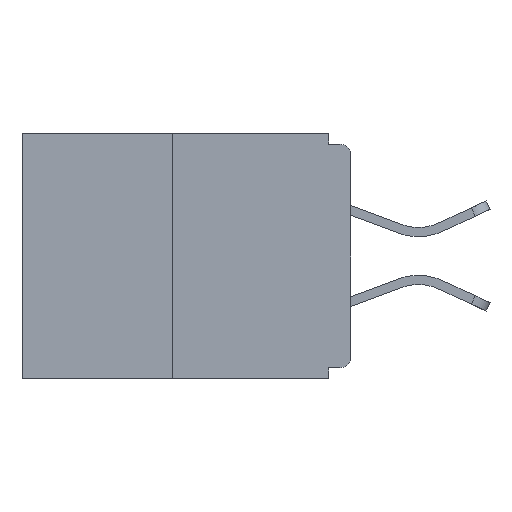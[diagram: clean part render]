
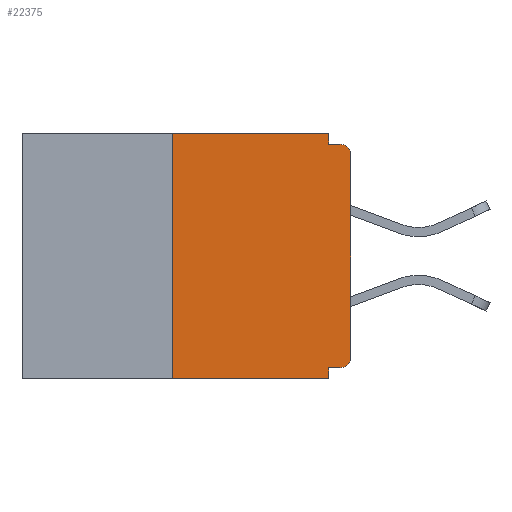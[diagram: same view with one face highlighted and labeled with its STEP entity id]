
A CAD part, left-side view. The second image highlights one B-rep face of the part: STEP entity #22375.
In plain terms, the highlighted planar face has unit normal (-1, 0, 0).
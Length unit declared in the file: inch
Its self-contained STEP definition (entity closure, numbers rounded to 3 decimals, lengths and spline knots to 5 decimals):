
#107 = DIRECTION ( 'NONE',  ( 0., -1., 0. ) ) ;
#208 = VERTEX_POINT ( 'NONE', #11022 ) ;
#245 = CARTESIAN_POINT ( 'NONE',  ( 0., 0.46, 0. ) ) ;
#309 = VERTEX_POINT ( 'NONE', #4111 ) ;
#477 = VECTOR ( 'NONE', #15684, 39.37008 ) ;
#879 = EDGE_CURVE ( 'NONE', #23807, #12587, #21511, .T. ) ;
#1698 = ORIENTED_EDGE ( 'NONE', *, *, #21080, .F. ) ;
#1701 = EDGE_CURVE ( 'NONE', #12587, #208, #19088, .T. ) ;
#1755 = VERTEX_POINT ( 'NONE', #23394 ) ;
#2341 = ORIENTED_EDGE ( 'NONE', *, *, #12382, .T. ) ;
#2353 = ORIENTED_EDGE ( 'NONE', *, *, #879, .T. ) ;
#2946 = VERTEX_POINT ( 'NONE', #4518 ) ;
#3126 = DIRECTION ( 'NONE',  ( 0., 0., -1. ) ) ;
#3643 = EDGE_CURVE ( 'NONE', #1755, #23119, #19013, .T. ) ;
#4021 = PLANE ( 'NONE',  #9224 ) ;
#4111 = CARTESIAN_POINT ( 'NONE',  ( 0., 0.25, -0.343 ) ) ;
#4428 = CARTESIAN_POINT ( 'NONE',  ( 0., 0.031, -0.015 ) ) ;
#4518 = CARTESIAN_POINT ( 'NONE',  ( 0., 0.031, -0.343 ) ) ;
#4547 = LINE ( 'NONE', #16645, #14903 ) ;
#4851 = DIRECTION ( 'NONE',  ( 0., 0., -1. ) ) ;
#5368 = VERTEX_POINT ( 'NONE', #4428 ) ;
#6048 = CARTESIAN_POINT ( 'NONE',  ( 0., 0.25, 0. ) ) ;
#6326 = ORIENTED_EDGE ( 'NONE', *, *, #9831, .T. ) ;
#6341 = CARTESIAN_POINT ( 'NONE',  ( 0., 0., -0.03 ) ) ;
#6537 = CARTESIAN_POINT ( 'NONE',  ( 0., 0.031, 0. ) ) ;
#6551 = CARTESIAN_POINT ( 'NONE',  ( 0., 0., 0. ) ) ;
#6879 = DIRECTION ( 'NONE',  ( 0., -1., 0. ) ) ;
#7056 = CARTESIAN_POINT ( 'NONE',  ( 0., 0.46, 0. ) ) ;
#7343 = FACE_OUTER_BOUND ( 'NONE', #18500, .T. ) ;
#8139 = CARTESIAN_POINT ( 'NONE',  ( 0., 0.015, -0.313 ) ) ;
#8490 = DIRECTION ( 'NONE',  ( 0., 1., 0. ) ) ;
#8572 = VECTOR ( 'NONE', #19128, 39.37008 ) ;
#8754 = DIRECTION ( 'NONE',  ( -1., 0., 0. ) ) ;
#8869 = ORIENTED_EDGE ( 'NONE', *, *, #17056, .F. ) ;
#9224 = AXIS2_PLACEMENT_3D ( 'NONE', #245, #20539, #13242 ) ;
#9308 = CARTESIAN_POINT ( 'NONE',  ( 0., 0.031, -0.343 ) ) ;
#9388 = VECTOR ( 'NONE', #18933, 39.37008 ) ;
#9685 = LINE ( 'NONE', #6048, #9388 ) ;
#9831 = EDGE_CURVE ( 'NONE', #1755, #23807, #16474, .T. ) ;
#10270 = CARTESIAN_POINT ( 'NONE',  ( 0., 0., -0.015 ) ) ;
#10283 = LINE ( 'NONE', #7056, #17644 ) ;
#11022 = CARTESIAN_POINT ( 'NONE',  ( 0., 0.015, -0.015 ) ) ;
#12271 = LINE ( 'NONE', #22230, #19795 ) ;
#12316 = DIRECTION ( 'NONE',  ( -1., 0., 0. ) ) ;
#12356 = ORIENTED_EDGE ( 'NONE', *, *, #14428, .F. ) ;
#12382 = EDGE_CURVE ( 'NONE', #309, #2946, #4547, .T. ) ;
#12587 = VERTEX_POINT ( 'NONE', #6341 ) ;
#13242 = DIRECTION ( 'NONE',  ( 0., 0., -1. ) ) ;
#14252 = LINE ( 'NONE', #10270, #477 ) ;
#14428 = EDGE_CURVE ( 'NONE', #23434, #15164, #10283, .T. ) ;
#14903 = VECTOR ( 'NONE', #107, 39.37008 ) ;
#15164 = VERTEX_POINT ( 'NONE', #6537 ) ;
#15374 = LINE ( 'NONE', #9308, #23443 ) ;
#15529 = CARTESIAN_POINT ( 'NONE',  ( 0., 0., -0.313 ) ) ;
#15684 = DIRECTION ( 'NONE',  ( 0., -1., 0. ) ) ;
#15887 = ORIENTED_EDGE ( 'NONE', *, *, #16235, .F. ) ;
#16235 = EDGE_CURVE ( 'NONE', #309, #23434, #9685, .T. ) ;
#16474 = CIRCLE ( 'NONE', #18007, 0.015 ) ;
#16645 = CARTESIAN_POINT ( 'NONE',  ( 0., 0.46, -0.343 ) ) ;
#17056 = EDGE_CURVE ( 'NONE', #5368, #208, #14252, .T. ) ;
#17334 = ORIENTED_EDGE ( 'NONE', *, *, #1701, .T. ) ;
#17565 = CARTESIAN_POINT ( 'NONE',  ( 0., 0.031, -0.328 ) ) ;
#17644 = VECTOR ( 'NONE', #6879, 39.37008 ) ;
#17996 = EDGE_CURVE ( 'NONE', #23119, #2946, #15374, .T. ) ;
#18007 = AXIS2_PLACEMENT_3D ( 'NONE', #8139, #12316, #4851 ) ;
#18066 = CARTESIAN_POINT ( 'NONE',  ( 0., 0.015, -0.03 ) ) ;
#18443 = DIRECTION ( 'NONE',  ( 0., 0., -1. ) ) ;
#18500 = EDGE_LOOP ( 'NONE', ( #12356, #15887, #2341, #21942, #20864, #6326, #2353, #17334, #8869, #1698 ) ) ;
#18933 = DIRECTION ( 'NONE',  ( 0., 0., 1. ) ) ;
#18946 = DIRECTION ( 'NONE',  ( 0., 0., -1. ) ) ;
#19013 = LINE ( 'NONE', #19506, #21586 ) ;
#19088 = CIRCLE ( 'NONE', #23761, 0.015 ) ;
#19128 = DIRECTION ( 'NONE',  ( 0., 0., 1. ) ) ;
#19506 = CARTESIAN_POINT ( 'NONE',  ( 0., 0., -0.328 ) ) ;
#19795 = VECTOR ( 'NONE', #18443, 39.37008 ) ;
#20539 = DIRECTION ( 'NONE',  ( 1., 0., 0. ) ) ;
#20864 = ORIENTED_EDGE ( 'NONE', *, *, #3643, .F. ) ;
#21080 = EDGE_CURVE ( 'NONE', #15164, #5368, #12271, .T. ) ;
#21511 = LINE ( 'NONE', #6551, #8572 ) ;
#21586 = VECTOR ( 'NONE', #8490, 39.37008 ) ;
#21916 = CARTESIAN_POINT ( 'NONE',  ( 0., 0.25, 0. ) ) ;
#21942 = ORIENTED_EDGE ( 'NONE', *, *, #17996, .F. ) ;
#22230 = CARTESIAN_POINT ( 'NONE',  ( 0., 0.031, 0. ) ) ;
#22375 = ADVANCED_FACE ( 'NONE', ( #7343 ), #4021, .F. ) ;
#23119 = VERTEX_POINT ( 'NONE', #17565 ) ;
#23394 = CARTESIAN_POINT ( 'NONE',  ( 0., 0.015, -0.328 ) ) ;
#23434 = VERTEX_POINT ( 'NONE', #21916 ) ;
#23443 = VECTOR ( 'NONE', #18946, 39.37008 ) ;
#23761 = AXIS2_PLACEMENT_3D ( 'NONE', #18066, #8754, #3126 ) ;
#23807 = VERTEX_POINT ( 'NONE', #15529 ) ;
